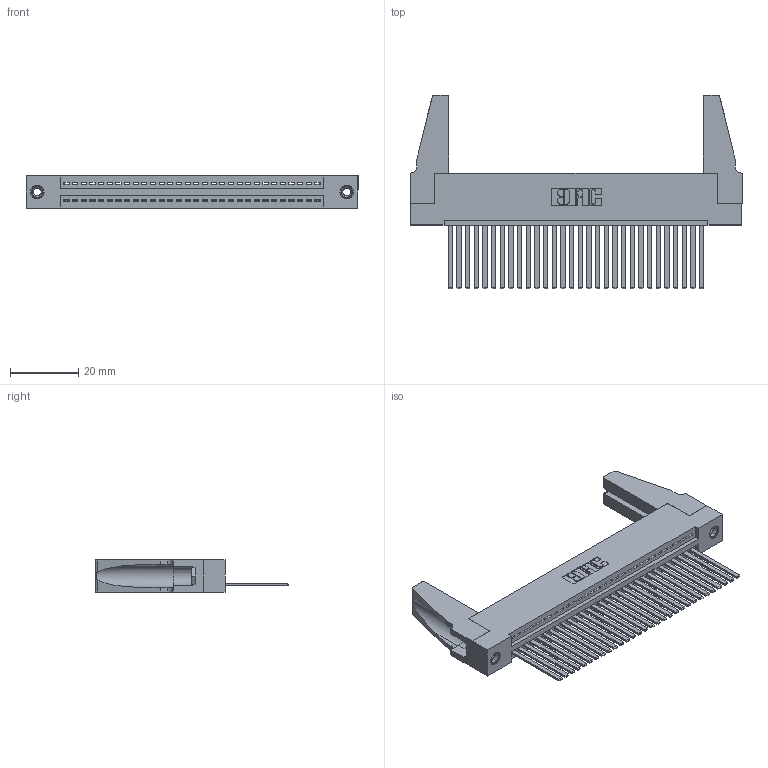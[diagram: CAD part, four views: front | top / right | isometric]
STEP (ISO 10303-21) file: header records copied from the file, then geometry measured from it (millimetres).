
FILE_DESCRIPTION (( 'STEP AP203' ), '1' );
FILE_NAME ('395-030-544-188.STEP', '2019-10-19T07:43:18', ( '' ), ( '' ), 'SwSTEP 2.0', 'SolidWorks 2016', '' );
FILE_SCHEMA (( 'CONFIG_CONTROL_DESIGN' ));
Length unit declared in the file: inch
Products named in the file (5): 345-220-078_345-220-088; 345 Part_Flush Mounting Lugs - 0.156 Dia-TH; 395-030-544-188; 345-292-001_345-293-144; 345-250-001_345-250-001-102
Assembly tree (35 placements, depth 2):
  395-030-544-188
    345 Part_Flush Mounting Lugs - 0.156 Dia-TH
    345-292-001_345-293-144  x30
    345-250-001_345-250-001-102  x2
    345-220-078_345-220-088  x2
Bounding box: 97.43 x 56.82 x 9.4 mm (x, y, z)
Volume: 12756.1 mm3; surface area: 16638.6 mm2
Topology: 35 solids, 35 shells, 1810 faces, 5395 edges, 3546 vertices
Faces by surface type: plane 1232, cylinder 562, cone 12, torus 4
Entity records: 26158 total; most frequent: CARTESIAN_POINT 4520, ORIENTED_EDGE 4444, DIRECTION 3970, EDGE_CURVE 2222, VECTOR 1932, LINE 1932, VERTEX_POINT 1474, AXIS2_PLACEMENT_3D 1019
